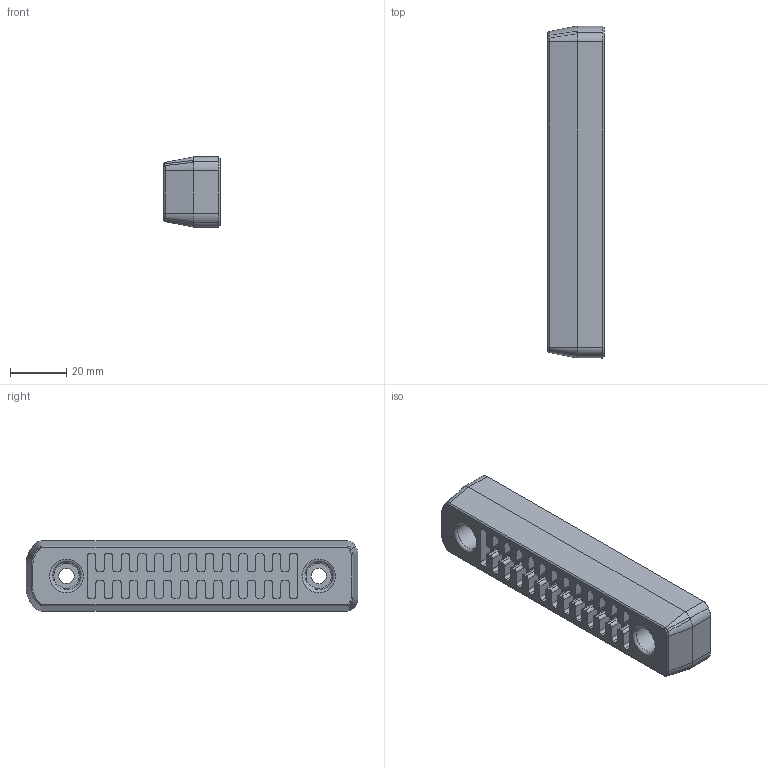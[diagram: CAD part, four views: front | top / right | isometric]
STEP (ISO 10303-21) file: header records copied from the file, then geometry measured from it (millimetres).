
FILE_DESCRIPTION (( 'STEP AP203' ), '1' );
FILE_NAME ('MOD9_G36_stock_butt-plate.STEP', '2020-07-07T01:45:33', ( '' ), ( '' ), 'SwSTEP 2.0', 'SolidWorks 2016', '' );
FILE_SCHEMA (( 'CONFIG_CONTROL_DESIGN' ));
Length unit declared in the file: millimetre
Products named in the file (1): MOD9_G36_stock_butt-plate
Bounding box: 19.99 x 118.4 x 25 mm (x, y, z)
Volume: 49372.9 mm3; surface area: 13953.8 mm2
Topology: 1 solids, 1 shells, 270 faces, 755 edges, 490 vertices
Faces by surface type: plane 121, cylinder 111, bspline 32, torus 4, cone 2
Full cylindrical faces by diameter (mm): 5.5 x2, 10 x2
Entity records: 9696 total; most frequent: CARTESIAN_POINT 2778, ORIENTED_EDGE 1486, DIRECTION 1365, EDGE_CURVE 743, VERTEX_POINT 488, LINE 463, VECTOR 463, AXIS2_PLACEMENT_3D 451
